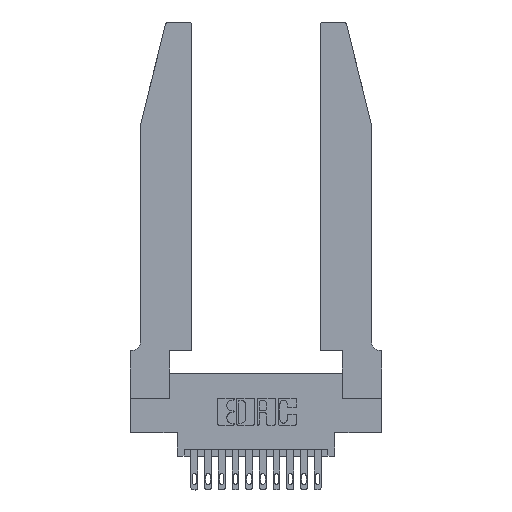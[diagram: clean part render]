
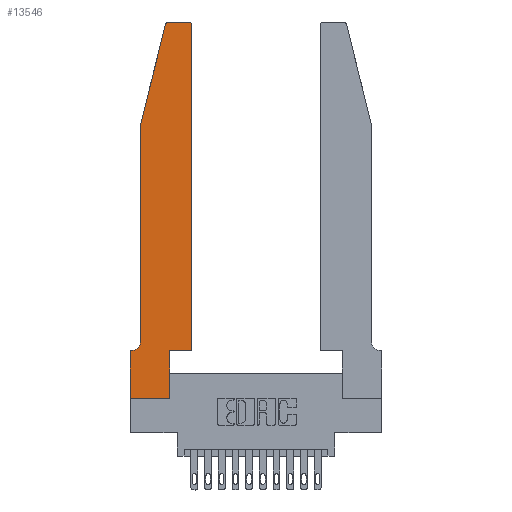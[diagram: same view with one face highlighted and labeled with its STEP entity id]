
A CAD part, top view. The second image highlights one B-rep face of the part: STEP entity #13546.
In plain terms, the highlighted planar face has unit normal (0, 0, 1).
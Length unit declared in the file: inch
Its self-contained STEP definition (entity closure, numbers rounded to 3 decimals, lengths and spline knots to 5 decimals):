
#325 = CARTESIAN_POINT ( 'NONE',  ( 0.0755, 2., 0.37 ) ) ;
#384 = DIRECTION ( 'NONE',  ( -1., 0., 0. ) ) ;
#601 = CARTESIAN_POINT ( 'NONE',  ( 0., 0., 0.37 ) ) ;
#631 = LINE ( 'NONE', #11246, #12138 ) ;
#634 = LINE ( 'NONE', #838, #1885 ) ;
#838 = CARTESIAN_POINT ( 'NONE',  ( 0.2605, 2.75, 0.37 ) ) ;
#890 = CARTESIAN_POINT ( 'NONE',  ( 0., 0.35, 0.37 ) ) ;
#1033 = VECTOR ( 'NONE', #7738, 39.37008 ) ;
#1077 = DIRECTION ( 'NONE',  ( 0., 1., 0. ) ) ;
#1125 = VECTOR ( 'NONE', #12157, 39.37008 ) ;
#1319 = VERTEX_POINT ( 'NONE', #9507 ) ;
#1326 = EDGE_CURVE ( 'NONE', #3998, #10458, #11528, .T. ) ;
#1658 = CARTESIAN_POINT ( 'NONE',  ( 0., 0., 0.37 ) ) ;
#1885 = VECTOR ( 'NONE', #8655, 39.37008 ) ;
#1901 = CARTESIAN_POINT ( 'NONE',  ( 0.0755, 2., 0.37 ) ) ;
#2437 = VECTOR ( 'NONE', #10843, 39.37008 ) ;
#2458 = CARTESIAN_POINT ( 'NONE',  ( 0.4505, 0.35, 0.37 ) ) ;
#2501 = DIRECTION ( 'NONE',  ( 0., 0., 1. ) ) ;
#2577 = ORIENTED_EDGE ( 'NONE', *, *, #2767, .T. ) ;
#2767 = EDGE_CURVE ( 'NONE', #1319, #8253, #631, .T. ) ;
#3209 = DIRECTION ( 'NONE',  ( 0., -1., 0. ) ) ;
#3250 = CARTESIAN_POINT ( 'NONE',  ( 0.4505, 2.72, 0.37 ) ) ;
#3313 = PLANE ( 'NONE',  #14875 ) ;
#3503 = VERTEX_POINT ( 'NONE', #6745 ) ;
#3528 = CARTESIAN_POINT ( 'NONE',  ( 0.4205, 2.75, 0.37 ) ) ;
#3882 = DIRECTION ( 'NONE',  ( 1., 0., 0. ) ) ;
#3939 = CARTESIAN_POINT ( 'NONE',  ( 0.4205, 2.72, 0.37 ) ) ;
#3998 = VERTEX_POINT ( 'NONE', #7800 ) ;
#4087 = ORIENTED_EDGE ( 'NONE', *, *, #12387, .T. ) ;
#4194 = EDGE_CURVE ( 'NONE', #8253, #12007, #5930, .T. ) ;
#4249 = CARTESIAN_POINT ( 'NONE',  ( 0.284, 2.72, 0.37 ) ) ;
#4626 = DIRECTION ( 'NONE',  ( 1., 0., 0. ) ) ;
#4741 = ORIENTED_EDGE ( 'NONE', *, *, #8494, .T. ) ;
#5107 = VERTEX_POINT ( 'NONE', #9480 ) ;
#5561 = CARTESIAN_POINT ( 'NONE',  ( 0.0055, 0.42, 0.37 ) ) ;
#5611 = EDGE_CURVE ( 'NONE', #8399, #11563, #5661, .T. ) ;
#5661 = CIRCLE ( 'NONE', #10116, 0.03 ) ;
#5729 = CIRCLE ( 'NONE', #8981, 0.03 ) ;
#5784 = CARTESIAN_POINT ( 'NONE',  ( 0., 0., 0.37 ) ) ;
#5930 = LINE ( 'NONE', #1901, #16768 ) ;
#5934 = LINE ( 'NONE', #1658, #2437 ) ;
#6105 = ORIENTED_EDGE ( 'NONE', *, *, #11318, .T. ) ;
#6335 = LINE ( 'NONE', #9196, #16995 ) ;
#6745 = CARTESIAN_POINT ( 'NONE',  ( 0.284, 2.75, 0.37 ) ) ;
#6900 = DIRECTION ( 'NONE',  ( -1., 0., 0. ) ) ;
#7738 = DIRECTION ( 'NONE',  ( 1., 0., 0. ) ) ;
#7800 = CARTESIAN_POINT ( 'NONE',  ( 0.0055, 0.35, 0.37 ) ) ;
#7806 = VERTEX_POINT ( 'NONE', #9900 ) ;
#8253 = VERTEX_POINT ( 'NONE', #325 ) ;
#8399 = VERTEX_POINT ( 'NONE', #3250 ) ;
#8494 = EDGE_CURVE ( 'NONE', #11563, #3503, #634, .T. ) ;
#8530 = FACE_OUTER_BOUND ( 'NONE', #10901, .T. ) ;
#8621 = ORIENTED_EDGE ( 'NONE', *, *, #13493, .T. ) ;
#8655 = DIRECTION ( 'NONE',  ( -1., 0., 0. ) ) ;
#8736 = ORIENTED_EDGE ( 'NONE', *, *, #8810, .T. ) ;
#8810 = EDGE_CURVE ( 'NONE', #7806, #15357, #13527, .T. ) ;
#8981 = AXIS2_PLACEMENT_3D ( 'NONE', #4249, #13455, #9671 ) ;
#9196 = CARTESIAN_POINT ( 'NONE',  ( 0.2865, 0.35, 0.37 ) ) ;
#9480 = CARTESIAN_POINT ( 'NONE',  ( 0.2865, 0., 0.37 ) ) ;
#9507 = CARTESIAN_POINT ( 'NONE',  ( 0.25487, 2.72718, 0.37 ) ) ;
#9671 = DIRECTION ( 'NONE',  ( 1., 0., 0. ) ) ;
#9804 = LINE ( 'NONE', #5784, #1125 ) ;
#9847 = AXIS2_PLACEMENT_3D ( 'NONE', #5561, #14720, #384 ) ;
#9900 = CARTESIAN_POINT ( 'NONE',  ( 0.2865, 0.35, 0.37 ) ) ;
#9903 = VERTEX_POINT ( 'NONE', #601 ) ;
#10116 = AXIS2_PLACEMENT_3D ( 'NONE', #3939, #2501, #3882 ) ;
#10154 = DIRECTION ( 'NONE',  ( -0.239, -0.971, 0. ) ) ;
#10225 = ORIENTED_EDGE ( 'NONE', *, *, #4194, .T. ) ;
#10313 = DIRECTION ( 'NONE',  ( 0., 1., 0. ) ) ;
#10458 = VERTEX_POINT ( 'NONE', #15592 ) ;
#10843 = DIRECTION ( 'NONE',  ( 0., -1., 0. ) ) ;
#10901 = EDGE_LOOP ( 'NONE', ( #4741, #14694, #2577, #10225, #6105, #15032, #11032, #8621, #16385, #8736, #4087, #15033 ) ) ;
#11032 = ORIENTED_EDGE ( 'NONE', *, *, #12098, .T. ) ;
#11246 = CARTESIAN_POINT ( 'NONE',  ( 0.0755, 2., 0.37 ) ) ;
#11318 = EDGE_CURVE ( 'NONE', #12007, #3998, #16932, .T. ) ;
#11453 = LINE ( 'NONE', #16814, #16559 ) ;
#11528 = LINE ( 'NONE', #14740, #16216 ) ;
#11563 = VERTEX_POINT ( 'NONE', #3528 ) ;
#12007 = VERTEX_POINT ( 'NONE', #15961 ) ;
#12098 = EDGE_CURVE ( 'NONE', #10458, #9903, #5934, .T. ) ;
#12138 = VECTOR ( 'NONE', #10154, 39.37008 ) ;
#12157 = DIRECTION ( 'NONE',  ( 1., 0., 0. ) ) ;
#12387 = EDGE_CURVE ( 'NONE', #15357, #8399, #11453, .T. ) ;
#12950 = CARTESIAN_POINT ( 'NONE',  ( 0.4505, 0.35, 0.37 ) ) ;
#13455 = DIRECTION ( 'NONE',  ( 0., 0., 1. ) ) ;
#13493 = EDGE_CURVE ( 'NONE', #9903, #5107, #9804, .T. ) ;
#13527 = LINE ( 'NONE', #12950, #1033 ) ;
#13546 = ADVANCED_FACE ( 'NONE', ( #8530 ), #3313, .T. ) ;
#14694 = ORIENTED_EDGE ( 'NONE', *, *, #14909, .T. ) ;
#14720 = DIRECTION ( 'NONE',  ( 0., 0., -1. ) ) ;
#14740 = CARTESIAN_POINT ( 'NONE',  ( 0.0755, 0.35, 0.37 ) ) ;
#14875 = AXIS2_PLACEMENT_3D ( 'NONE', #890, #15041, #4626 ) ;
#14909 = EDGE_CURVE ( 'NONE', #3503, #1319, #5729, .T. ) ;
#15032 = ORIENTED_EDGE ( 'NONE', *, *, #1326, .T. ) ;
#15033 = ORIENTED_EDGE ( 'NONE', *, *, #5611, .T. ) ;
#15041 = DIRECTION ( 'NONE',  ( 0., 0., 1. ) ) ;
#15255 = EDGE_CURVE ( 'NONE', #5107, #7806, #6335, .T. ) ;
#15357 = VERTEX_POINT ( 'NONE', #2458 ) ;
#15592 = CARTESIAN_POINT ( 'NONE',  ( 0., 0.35, 0.37 ) ) ;
#15961 = CARTESIAN_POINT ( 'NONE',  ( 0.0755, 0.42, 0.37 ) ) ;
#16216 = VECTOR ( 'NONE', #6900, 39.37008 ) ;
#16385 = ORIENTED_EDGE ( 'NONE', *, *, #15255, .T. ) ;
#16559 = VECTOR ( 'NONE', #10313, 39.37008 ) ;
#16768 = VECTOR ( 'NONE', #3209, 39.37008 ) ;
#16814 = CARTESIAN_POINT ( 'NONE',  ( 0.4505, 0.35, 0.37 ) ) ;
#16932 = CIRCLE ( 'NONE', #9847, 0.07 ) ;
#16995 = VECTOR ( 'NONE', #1077, 39.37008 ) ;
